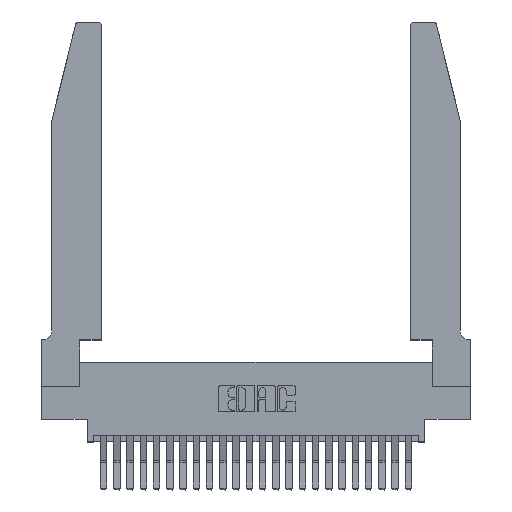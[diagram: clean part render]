
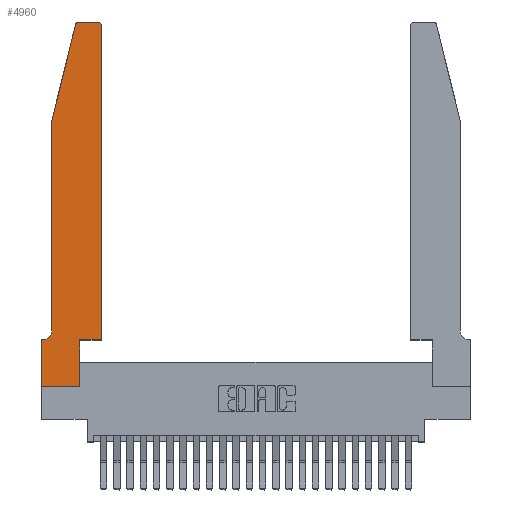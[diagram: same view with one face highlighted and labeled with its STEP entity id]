
A CAD part, top view. The second image highlights one B-rep face of the part: STEP entity #4960.
In plain terms, the highlighted planar face has unit normal (0, 0, 1).
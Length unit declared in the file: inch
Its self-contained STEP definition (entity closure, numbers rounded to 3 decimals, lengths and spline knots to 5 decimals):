
#403 = VERTEX_POINT ( 'NONE', #24842 ) ;
#749 = VECTOR ( 'NONE', #20094, 39.37008 ) ;
#918 = CARTESIAN_POINT ( 'NONE',  ( 0.4205, 2.75, 0.37 ) ) ;
#936 = ORIENTED_EDGE ( 'NONE', *, *, #8010, .T. ) ;
#1117 = EDGE_CURVE ( 'NONE', #14688, #5114, #20897, .T. ) ;
#1407 = VERTEX_POINT ( 'NONE', #18962 ) ;
#1587 = ORIENTED_EDGE ( 'NONE', *, *, #24832, .T. ) ;
#1777 = EDGE_CURVE ( 'NONE', #7563, #16593, #17685, .T. ) ;
#1809 = VERTEX_POINT ( 'NONE', #15839 ) ;
#2305 = CARTESIAN_POINT ( 'NONE',  ( 0.2865, 0.35, 0.37 ) ) ;
#2605 = EDGE_CURVE ( 'NONE', #1809, #9501, #4059, .T. ) ;
#2867 = CARTESIAN_POINT ( 'NONE',  ( 0.2605, 2.75, 0.37 ) ) ;
#3377 = DIRECTION ( 'NONE',  ( 0., 0., 1. ) ) ;
#3431 = DIRECTION ( 'NONE',  ( -0.239, -0.971, 0. ) ) ;
#3655 = EDGE_CURVE ( 'NONE', #9501, #403, #13767, .T. ) ;
#3724 = ORIENTED_EDGE ( 'NONE', *, *, #2605, .T. ) ;
#3813 = CARTESIAN_POINT ( 'NONE',  ( 0.0755, 2., 0.37 ) ) ;
#4059 = LINE ( 'NONE', #2305, #18896 ) ;
#4696 = AXIS2_PLACEMENT_3D ( 'NONE', #26109, #5960, #13944 ) ;
#4960 = ADVANCED_FACE ( 'NONE', ( #9986 ), #11924, .T. ) ;
#5114 = VERTEX_POINT ( 'NONE', #24603 ) ;
#5214 = VERTEX_POINT ( 'NONE', #10762 ) ;
#5326 = CARTESIAN_POINT ( 'NONE',  ( 0.4205, 2.72, 0.37 ) ) ;
#5592 = VECTOR ( 'NONE', #8224, 39.37008 ) ;
#5960 = DIRECTION ( 'NONE',  ( 0., 0., 1. ) ) ;
#6161 = CARTESIAN_POINT ( 'NONE',  ( 0.0755, 0.35, 0.37 ) ) ;
#6173 = ORIENTED_EDGE ( 'NONE', *, *, #20251, .T. ) ;
#6272 = ORIENTED_EDGE ( 'NONE', *, *, #1777, .T. ) ;
#6977 = LINE ( 'NONE', #21560, #15169 ) ;
#6987 = DIRECTION ( 'NONE',  ( -1., 0., 0. ) ) ;
#7134 = CARTESIAN_POINT ( 'NONE',  ( 0.2865, 0.35, 0.37 ) ) ;
#7563 = VERTEX_POINT ( 'NONE', #918 ) ;
#7662 = ORIENTED_EDGE ( 'NONE', *, *, #1117, .T. ) ;
#7729 = DIRECTION ( 'NONE',  ( 0., -1., 0. ) ) ;
#7899 = ORIENTED_EDGE ( 'NONE', *, *, #12946, .T. ) ;
#8010 = EDGE_CURVE ( 'NONE', #12769, #9349, #25876, .T. ) ;
#8224 = DIRECTION ( 'NONE',  ( 1., 0., 0. ) ) ;
#8891 = EDGE_CURVE ( 'NONE', #5114, #12769, #16981, .T. ) ;
#9144 = DIRECTION ( 'NONE',  ( 0., 0., 1. ) ) ;
#9349 = VERTEX_POINT ( 'NONE', #24480 ) ;
#9501 = VERTEX_POINT ( 'NONE', #7134 ) ;
#9540 = DIRECTION ( 'NONE',  ( 1., 0., 0. ) ) ;
#9986 = FACE_OUTER_BOUND ( 'NONE', #24542, .T. ) ;
#10070 = EDGE_CURVE ( 'NONE', #5214, #7563, #10916, .T. ) ;
#10762 = CARTESIAN_POINT ( 'NONE',  ( 0.4505, 2.72, 0.37 ) ) ;
#10916 = CIRCLE ( 'NONE', #11020, 0.03 ) ;
#11020 = AXIS2_PLACEMENT_3D ( 'NONE', #5326, #3377, #9540 ) ;
#11171 = DIRECTION ( 'NONE',  ( 1., 0., 0. ) ) ;
#11423 = CARTESIAN_POINT ( 'NONE',  ( 0., 0., 0.37 ) ) ;
#11510 = LINE ( 'NONE', #12306, #749 ) ;
#11783 = CIRCLE ( 'NONE', #14497, 0.03 ) ;
#11924 = PLANE ( 'NONE',  #4696 ) ;
#12032 = ORIENTED_EDGE ( 'NONE', *, *, #10070, .T. ) ;
#12241 = VECTOR ( 'NONE', #20271, 39.37008 ) ;
#12306 = CARTESIAN_POINT ( 'NONE',  ( 0., 0., 0.37 ) ) ;
#12411 = CARTESIAN_POINT ( 'NONE',  ( 0.0755, 2., 0.37 ) ) ;
#12769 = VERTEX_POINT ( 'NONE', #24035 ) ;
#12946 = EDGE_CURVE ( 'NONE', #1407, #1809, #11510, .T. ) ;
#13164 = DIRECTION ( 'NONE',  ( 0., 1., 0. ) ) ;
#13303 = LINE ( 'NONE', #11423, #21212 ) ;
#13767 = LINE ( 'NONE', #17070, #5592 ) ;
#13779 = LINE ( 'NONE', #19242, #16650 ) ;
#13944 = DIRECTION ( 'NONE',  ( 1., 0., 0. ) ) ;
#14497 = AXIS2_PLACEMENT_3D ( 'NONE', #25430, #9144, #11171 ) ;
#14518 = VECTOR ( 'NONE', #21084, 39.37008 ) ;
#14688 = VERTEX_POINT ( 'NONE', #12411 ) ;
#14849 = CARTESIAN_POINT ( 'NONE',  ( 0.25487, 2.72718, 0.37 ) ) ;
#14976 = CARTESIAN_POINT ( 'NONE',  ( 0.284, 2.75, 0.37 ) ) ;
#15169 = VECTOR ( 'NONE', #13164, 39.37008 ) ;
#15839 = CARTESIAN_POINT ( 'NONE',  ( 0.2865, 0., 0.37 ) ) ;
#15906 = EDGE_CURVE ( 'NONE', #403, #5214, #6977, .T. ) ;
#16593 = VERTEX_POINT ( 'NONE', #14976 ) ;
#16650 = VECTOR ( 'NONE', #3431, 39.37008 ) ;
#16981 = CIRCLE ( 'NONE', #24925, 0.07 ) ;
#17070 = CARTESIAN_POINT ( 'NONE',  ( 0.4505, 0.35, 0.37 ) ) ;
#17087 = VECTOR ( 'NONE', #19808, 39.37008 ) ;
#17163 = ORIENTED_EDGE ( 'NONE', *, *, #8891, .T. ) ;
#17685 = LINE ( 'NONE', #2867, #14518 ) ;
#18536 = EDGE_CURVE ( 'NONE', #9349, #1407, #13303, .T. ) ;
#18896 = VECTOR ( 'NONE', #22494, 39.37008 ) ;
#18962 = CARTESIAN_POINT ( 'NONE',  ( 0., 0., 0.37 ) ) ;
#19242 = CARTESIAN_POINT ( 'NONE',  ( 0.0755, 2., 0.37 ) ) ;
#19808 = DIRECTION ( 'NONE',  ( 0., -1., 0. ) ) ;
#20094 = DIRECTION ( 'NONE',  ( 1., 0., 0. ) ) ;
#20251 = EDGE_CURVE ( 'NONE', #16593, #24088, #11783, .T. ) ;
#20271 = DIRECTION ( 'NONE',  ( -1., 0., 0. ) ) ;
#20581 = ORIENTED_EDGE ( 'NONE', *, *, #18536, .T. ) ;
#20897 = LINE ( 'NONE', #3813, #17087 ) ;
#21084 = DIRECTION ( 'NONE',  ( -1., 0., 0. ) ) ;
#21127 = CARTESIAN_POINT ( 'NONE',  ( 0.0055, 0.42, 0.37 ) ) ;
#21212 = VECTOR ( 'NONE', #7729, 39.37008 ) ;
#21560 = CARTESIAN_POINT ( 'NONE',  ( 0.4505, 0.35, 0.37 ) ) ;
#21967 = ORIENTED_EDGE ( 'NONE', *, *, #3655, .T. ) ;
#22494 = DIRECTION ( 'NONE',  ( 0., 1., 0. ) ) ;
#24035 = CARTESIAN_POINT ( 'NONE',  ( 0.0055, 0.35, 0.37 ) ) ;
#24088 = VERTEX_POINT ( 'NONE', #14849 ) ;
#24230 = ORIENTED_EDGE ( 'NONE', *, *, #15906, .T. ) ;
#24480 = CARTESIAN_POINT ( 'NONE',  ( 0., 0.35, 0.37 ) ) ;
#24542 = EDGE_LOOP ( 'NONE', ( #6272, #6173, #1587, #7662, #17163, #936, #20581, #7899, #3724, #21967, #24230, #12032 ) ) ;
#24603 = CARTESIAN_POINT ( 'NONE',  ( 0.0755, 0.42, 0.37 ) ) ;
#24832 = EDGE_CURVE ( 'NONE', #24088, #14688, #13779, .T. ) ;
#24842 = CARTESIAN_POINT ( 'NONE',  ( 0.4505, 0.35, 0.37 ) ) ;
#24925 = AXIS2_PLACEMENT_3D ( 'NONE', #21127, #25553, #6987 ) ;
#25430 = CARTESIAN_POINT ( 'NONE',  ( 0.284, 2.72, 0.37 ) ) ;
#25553 = DIRECTION ( 'NONE',  ( 0., 0., -1. ) ) ;
#25876 = LINE ( 'NONE', #6161, #12241 ) ;
#26109 = CARTESIAN_POINT ( 'NONE',  ( 0., 0.35, 0.37 ) ) ;
